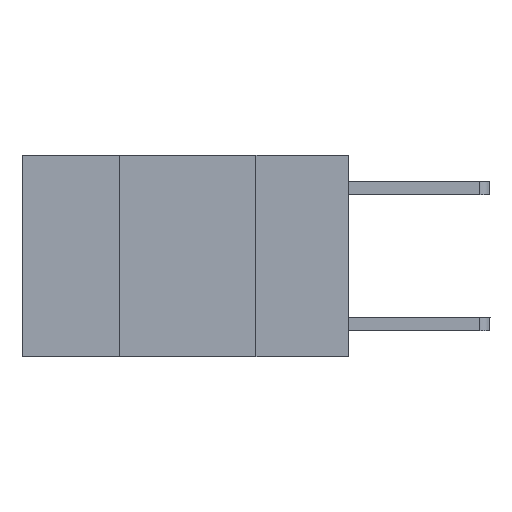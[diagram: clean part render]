
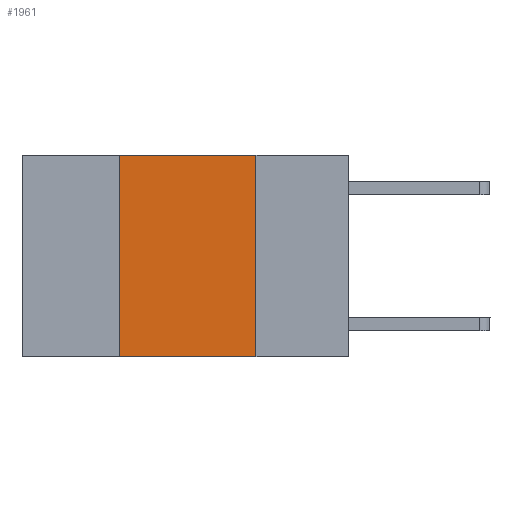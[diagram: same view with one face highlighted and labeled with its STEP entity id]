
A CAD part, left-side view. The second image highlights one B-rep face of the part: STEP entity #1961.
In plain terms, the highlighted planar face has unit normal (-1, 0, 0).
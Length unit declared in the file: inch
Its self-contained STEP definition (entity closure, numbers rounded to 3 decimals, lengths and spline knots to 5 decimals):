
#98 = CARTESIAN_POINT ( 'NONE',  ( 0., 0.6, 0. ) ) ;
#150 = LINE ( 'NONE', #4372, #6778 ) ;
#377 = LINE ( 'NONE', #2419, #4716 ) ;
#523 = DIRECTION ( 'NONE',  ( 0., 0., -1. ) ) ;
#767 = VECTOR ( 'NONE', #523, 39.37008 ) ;
#1122 = CARTESIAN_POINT ( 'NONE',  ( 0., 0.17, 0. ) ) ;
#1236 = CARTESIAN_POINT ( 'NONE',  ( 0., 0.42, 0. ) ) ;
#1373 = PLANE ( 'NONE',  #2289 ) ;
#1379 = EDGE_LOOP ( 'NONE', ( #6689, #8176, #7789, #4651 ) ) ;
#1480 = DIRECTION ( 'NONE',  ( 0., 0., 1. ) ) ;
#1860 = VERTEX_POINT ( 'NONE', #1122 ) ;
#1961 = ADVANCED_FACE ( 'NONE', ( #3794 ), #1373, .F. ) ;
#2289 = AXIS2_PLACEMENT_3D ( 'NONE', #5631, #3129, #2310 ) ;
#2300 = EDGE_CURVE ( 'NONE', #9296, #1860, #6246, .T. ) ;
#2310 = DIRECTION ( 'NONE',  ( 0., 0., -1. ) ) ;
#2399 = VERTEX_POINT ( 'NONE', #6273 ) ;
#2419 = CARTESIAN_POINT ( 'NONE',  ( 0., 0.42, 0. ) ) ;
#2843 = DIRECTION ( 'NONE',  ( 0., -1., 0. ) ) ;
#3129 = DIRECTION ( 'NONE',  ( 1., 0., 0. ) ) ;
#3794 = FACE_OUTER_BOUND ( 'NONE', #1379, .T. ) ;
#4024 = VECTOR ( 'NONE', #2843, 39.37008 ) ;
#4132 = EDGE_CURVE ( 'NONE', #1860, #2399, #7915, .T. ) ;
#4372 = CARTESIAN_POINT ( 'NONE',  ( 0., 0.6, -0.37 ) ) ;
#4651 = ORIENTED_EDGE ( 'NONE', *, *, #7031, .T. ) ;
#4716 = VECTOR ( 'NONE', #1480, 39.37008 ) ;
#4759 = EDGE_CURVE ( 'NONE', #5257, #9296, #377, .T. ) ;
#5257 = VERTEX_POINT ( 'NONE', #7305 ) ;
#5631 = CARTESIAN_POINT ( 'NONE',  ( 0., 0.6, 0. ) ) ;
#6246 = LINE ( 'NONE', #98, #4024 ) ;
#6273 = CARTESIAN_POINT ( 'NONE',  ( 0., 0.17, -0.37 ) ) ;
#6689 = ORIENTED_EDGE ( 'NONE', *, *, #4132, .F. ) ;
#6778 = VECTOR ( 'NONE', #7800, 39.37008 ) ;
#7031 = EDGE_CURVE ( 'NONE', #5257, #2399, #150, .T. ) ;
#7305 = CARTESIAN_POINT ( 'NONE',  ( 0., 0.42, -0.37 ) ) ;
#7789 = ORIENTED_EDGE ( 'NONE', *, *, #4759, .F. ) ;
#7800 = DIRECTION ( 'NONE',  ( 0., -1., 0. ) ) ;
#7915 = LINE ( 'NONE', #9089, #767 ) ;
#8176 = ORIENTED_EDGE ( 'NONE', *, *, #2300, .F. ) ;
#9089 = CARTESIAN_POINT ( 'NONE',  ( 0., 0.17, 0. ) ) ;
#9296 = VERTEX_POINT ( 'NONE', #1236 ) ;
